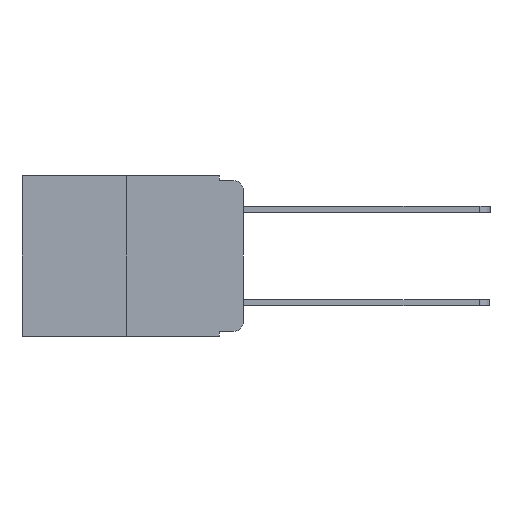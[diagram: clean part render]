
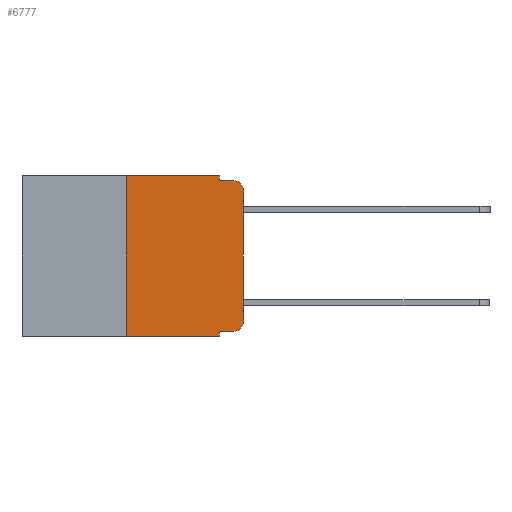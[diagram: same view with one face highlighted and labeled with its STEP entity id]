
A CAD part, left-side view. The second image highlights one B-rep face of the part: STEP entity #6777.
In plain terms, the highlighted planar face has unit normal (-1, 0, 0).
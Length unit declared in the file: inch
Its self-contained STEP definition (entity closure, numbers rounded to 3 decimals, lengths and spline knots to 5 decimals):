
#80 = VERTEX_POINT ( 'NONE', #12573 ) ;
#428 = CIRCLE ( 'NONE', #764, 0.02 ) ;
#465 = CARTESIAN_POINT ( 'NONE',  ( 0., 0.02, -0.01 ) ) ;
#534 = CARTESIAN_POINT ( 'NONE',  ( 0., 0.02, -0.333 ) ) ;
#548 = ORIENTED_EDGE ( 'NONE', *, *, #12098, .F. ) ;
#581 = CARTESIAN_POINT ( 'NONE',  ( 0., 0.473, 0. ) ) ;
#668 = DIRECTION ( 'NONE',  ( 1., 0., 0. ) ) ;
#752 = ORIENTED_EDGE ( 'NONE', *, *, #17787, .T. ) ;
#764 = AXIS2_PLACEMENT_3D ( 'NONE', #11150, #15956, #15872 ) ;
#1052 = EDGE_CURVE ( 'NONE', #17018, #5342, #13293, .T. ) ;
#1173 = LINE ( 'NONE', #18809, #15831 ) ;
#1246 = CARTESIAN_POINT ( 'NONE',  ( 0., 0., -0.03 ) ) ;
#1341 = EDGE_CURVE ( 'NONE', #5342, #80, #12355, .T. ) ;
#1452 = ORIENTED_EDGE ( 'NONE', *, *, #18642, .T. ) ;
#1790 = ORIENTED_EDGE ( 'NONE', *, *, #6288, .T. ) ;
#1794 = FACE_OUTER_BOUND ( 'NONE', #20932, .T. ) ;
#1837 = EDGE_CURVE ( 'NONE', #21132, #10813, #428, .T. ) ;
#1937 = LINE ( 'NONE', #8325, #18380 ) ;
#2015 = VECTOR ( 'NONE', #7785, 39.37008 ) ;
#2961 = ORIENTED_EDGE ( 'NONE', *, *, #16688, .T. ) ;
#3107 = CARTESIAN_POINT ( 'NONE',  ( 0., 0.02, -0.03 ) ) ;
#3306 = CARTESIAN_POINT ( 'NONE',  ( 0., 0.051, 0. ) ) ;
#4424 = CARTESIAN_POINT ( 'NONE',  ( 0., 0.25, 0. ) ) ;
#5161 = DIRECTION ( 'NONE',  ( 0., 0., -1. ) ) ;
#5342 = VERTEX_POINT ( 'NONE', #3306 ) ;
#5840 = VECTOR ( 'NONE', #18386, 39.37008 ) ;
#6069 = LINE ( 'NONE', #9772, #15939 ) ;
#6288 = EDGE_CURVE ( 'NONE', #10813, #16693, #24512, .T. ) ;
#6682 = ORIENTED_EDGE ( 'NONE', *, *, #1052, .F. ) ;
#6777 = ADVANCED_FACE ( 'NONE', ( #1794 ), #24185, .F. ) ;
#6951 = VERTEX_POINT ( 'NONE', #7133 ) ;
#7133 = CARTESIAN_POINT ( 'NONE',  ( 0., 0.051, -0.343 ) ) ;
#7785 = DIRECTION ( 'NONE',  ( 0., -1., 0. ) ) ;
#8325 = CARTESIAN_POINT ( 'NONE',  ( 0., 0.051, -0.01 ) ) ;
#8466 = VERTEX_POINT ( 'NONE', #21645 ) ;
#8810 = ORIENTED_EDGE ( 'NONE', *, *, #1341, .F. ) ;
#9071 = DIRECTION ( 'NONE',  ( 0., 0., 1. ) ) ;
#9583 = ORIENTED_EDGE ( 'NONE', *, *, #12593, .F. ) ;
#9772 = CARTESIAN_POINT ( 'NONE',  ( 0., 0.051, 0. ) ) ;
#9875 = DIRECTION ( 'NONE',  ( 0., -1., 0. ) ) ;
#10813 = VERTEX_POINT ( 'NONE', #12503 ) ;
#10930 = LINE ( 'NONE', #22062, #20667 ) ;
#11150 = CARTESIAN_POINT ( 'NONE',  ( 0., 0.02, -0.313 ) ) ;
#11353 = DIRECTION ( 'NONE',  ( 0., -1., 0. ) ) ;
#12098 = EDGE_CURVE ( 'NONE', #80, #21911, #1937, .T. ) ;
#12345 = ORIENTED_EDGE ( 'NONE', *, *, #22928, .F. ) ;
#12355 = LINE ( 'NONE', #24639, #5840 ) ;
#12503 = CARTESIAN_POINT ( 'NONE',  ( 0., 0., -0.313 ) ) ;
#12573 = CARTESIAN_POINT ( 'NONE',  ( 0., 0.051, -0.01 ) ) ;
#12593 = EDGE_CURVE ( 'NONE', #22605, #6951, #6069, .T. ) ;
#13103 = VECTOR ( 'NONE', #24622, 39.37008 ) ;
#13293 = LINE ( 'NONE', #21188, #2015 ) ;
#14655 = DIRECTION ( 'NONE',  ( 0., 0., -1. ) ) ;
#15613 = DIRECTION ( 'NONE',  ( 0., 0., -1. ) ) ;
#15831 = VECTOR ( 'NONE', #9071, 39.37008 ) ;
#15872 = DIRECTION ( 'NONE',  ( 0., 0., -1. ) ) ;
#15939 = VECTOR ( 'NONE', #15613, 39.37008 ) ;
#15956 = DIRECTION ( 'NONE',  ( -1., 0., 0. ) ) ;
#16482 = VECTOR ( 'NONE', #11353, 39.37008 ) ;
#16688 = EDGE_CURVE ( 'NONE', #8466, #6951, #25403, .T. ) ;
#16693 = VERTEX_POINT ( 'NONE', #1246 ) ;
#16959 = CARTESIAN_POINT ( 'NONE',  ( 0., 0., 0. ) ) ;
#16967 = DIRECTION ( 'NONE',  ( -1., 0., 0. ) ) ;
#17018 = VERTEX_POINT ( 'NONE', #4424 ) ;
#17618 = CIRCLE ( 'NONE', #20899, 0.02 ) ;
#17787 = EDGE_CURVE ( 'NONE', #22605, #21132, #10930, .T. ) ;
#18380 = VECTOR ( 'NONE', #9875, 39.37008 ) ;
#18386 = DIRECTION ( 'NONE',  ( 0., 0., -1. ) ) ;
#18642 = EDGE_CURVE ( 'NONE', #16693, #21911, #17618, .T. ) ;
#18809 = CARTESIAN_POINT ( 'NONE',  ( 0., 0.25, 0. ) ) ;
#20667 = VECTOR ( 'NONE', #23934, 39.37008 ) ;
#20899 = AXIS2_PLACEMENT_3D ( 'NONE', #3107, #16967, #5161 ) ;
#20932 = EDGE_LOOP ( 'NONE', ( #1790, #1452, #548, #8810, #6682, #12345, #2961, #9583, #752, #23480 ) ) ;
#21132 = VERTEX_POINT ( 'NONE', #534 ) ;
#21188 = CARTESIAN_POINT ( 'NONE',  ( 0., 0.473, 0. ) ) ;
#21645 = CARTESIAN_POINT ( 'NONE',  ( 0., 0.25, -0.343 ) ) ;
#21911 = VERTEX_POINT ( 'NONE', #465 ) ;
#22062 = CARTESIAN_POINT ( 'NONE',  ( 0., 0.051, -0.333 ) ) ;
#22452 = AXIS2_PLACEMENT_3D ( 'NONE', #581, #668, #14655 ) ;
#22605 = VERTEX_POINT ( 'NONE', #22766 ) ;
#22766 = CARTESIAN_POINT ( 'NONE',  ( 0., 0.051, -0.333 ) ) ;
#22921 = CARTESIAN_POINT ( 'NONE',  ( 0., 0.473, -0.343 ) ) ;
#22928 = EDGE_CURVE ( 'NONE', #8466, #17018, #1173, .T. ) ;
#23480 = ORIENTED_EDGE ( 'NONE', *, *, #1837, .T. ) ;
#23934 = DIRECTION ( 'NONE',  ( 0., -1., 0. ) ) ;
#24185 = PLANE ( 'NONE',  #22452 ) ;
#24512 = LINE ( 'NONE', #16959, #13103 ) ;
#24622 = DIRECTION ( 'NONE',  ( 0., 0., 1. ) ) ;
#24639 = CARTESIAN_POINT ( 'NONE',  ( 0., 0.051, 0. ) ) ;
#25403 = LINE ( 'NONE', #22921, #16482 ) ;
